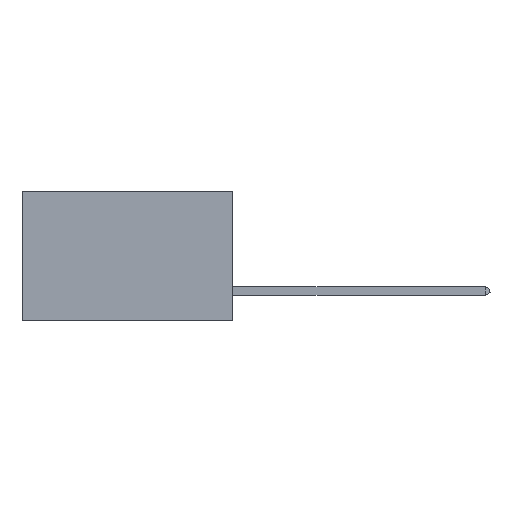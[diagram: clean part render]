
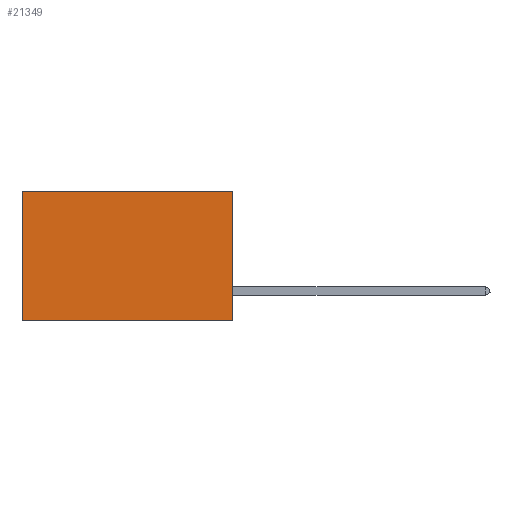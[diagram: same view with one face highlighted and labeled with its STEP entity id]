
A CAD part, left-side view. The second image highlights one B-rep face of the part: STEP entity #21349.
In plain terms, the highlighted planar face has unit normal (-1, 0, 0).
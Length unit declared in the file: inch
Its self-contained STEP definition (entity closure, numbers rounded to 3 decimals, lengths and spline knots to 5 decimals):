
#1496 = LINE ( 'NONE', #23052, #11082 ) ;
#2076 = VERTEX_POINT ( 'NONE', #4007 ) ;
#2562 = DIRECTION ( 'NONE',  ( 0., 0., -1. ) ) ;
#3378 = VECTOR ( 'NONE', #28311, 39.37008 ) ;
#4007 = CARTESIAN_POINT ( 'NONE',  ( 0.2875, 0., -0.37 ) ) ;
#5153 = EDGE_CURVE ( 'NONE', #18547, #19051, #10590, .T. ) ;
#6143 = CARTESIAN_POINT ( 'NONE',  ( 0.2875, 0., 0. ) ) ;
#7353 = ORIENTED_EDGE ( 'NONE', *, *, #8252, .F. ) ;
#8252 = EDGE_CURVE ( 'NONE', #32268, #2076, #29215, .T. ) ;
#8388 = EDGE_CURVE ( 'NONE', #32268, #18547, #21795, .T. ) ;
#10590 = LINE ( 'NONE', #19373, #34731 ) ;
#11082 = VECTOR ( 'NONE', #11985, 39.37008 ) ;
#11985 = DIRECTION ( 'NONE',  ( 0., 1., 0. ) ) ;
#12415 = CARTESIAN_POINT ( 'NONE',  ( 0.2875, 0.6, -0.37 ) ) ;
#13130 = CARTESIAN_POINT ( 'NONE',  ( 0.2875, 0., 0. ) ) ;
#13234 = PLANE ( 'NONE',  #17230 ) ;
#13926 = VECTOR ( 'NONE', #33469, 39.37008 ) ;
#16819 = ORIENTED_EDGE ( 'NONE', *, *, #5153, .T. ) ;
#17230 = AXIS2_PLACEMENT_3D ( 'NONE', #21692, #35276, #26925 ) ;
#18304 = EDGE_CURVE ( 'NONE', #2076, #19051, #1496, .T. ) ;
#18547 = VERTEX_POINT ( 'NONE', #20659 ) ;
#19051 = VERTEX_POINT ( 'NONE', #12415 ) ;
#19373 = CARTESIAN_POINT ( 'NONE',  ( 0.2875, 0.6, 0. ) ) ;
#20659 = CARTESIAN_POINT ( 'NONE',  ( 0.2875, 0.6, 0. ) ) ;
#21349 = ADVANCED_FACE ( 'NONE', ( #22395 ), #13234, .F. ) ;
#21692 = CARTESIAN_POINT ( 'NONE',  ( 0.2875, 0., 0. ) ) ;
#21795 = LINE ( 'NONE', #6143, #3378 ) ;
#22037 = CARTESIAN_POINT ( 'NONE',  ( 0.2875, 0., 0. ) ) ;
#22395 = FACE_OUTER_BOUND ( 'NONE', #33917, .T. ) ;
#22799 = ORIENTED_EDGE ( 'NONE', *, *, #18304, .F. ) ;
#23052 = CARTESIAN_POINT ( 'NONE',  ( 0.2875, 0., -0.37 ) ) ;
#24058 = ORIENTED_EDGE ( 'NONE', *, *, #8388, .T. ) ;
#26925 = DIRECTION ( 'NONE',  ( 0., 0., -1. ) ) ;
#28311 = DIRECTION ( 'NONE',  ( 0., 1., 0. ) ) ;
#29215 = LINE ( 'NONE', #13130, #13926 ) ;
#32268 = VERTEX_POINT ( 'NONE', #22037 ) ;
#33469 = DIRECTION ( 'NONE',  ( 0., 0., -1. ) ) ;
#33917 = EDGE_LOOP ( 'NONE', ( #16819, #22799, #7353, #24058 ) ) ;
#34731 = VECTOR ( 'NONE', #2562, 39.37008 ) ;
#35276 = DIRECTION ( 'NONE',  ( 1., 0., 0. ) ) ;
